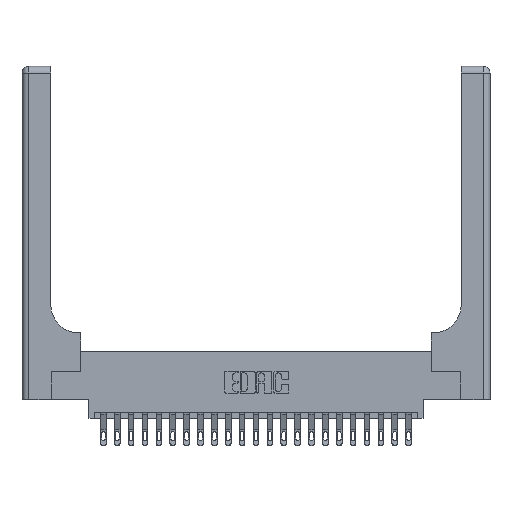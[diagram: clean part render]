
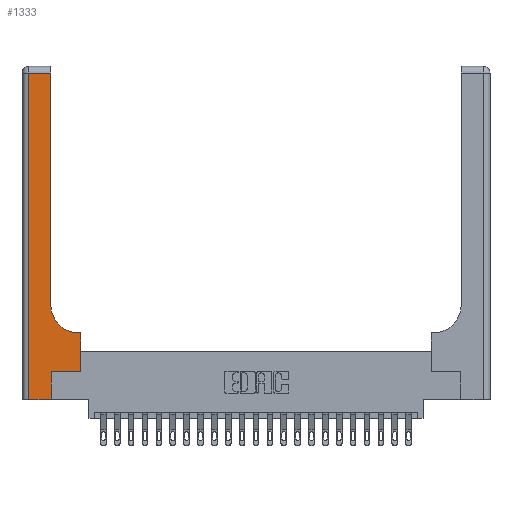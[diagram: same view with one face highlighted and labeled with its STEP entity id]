
A CAD part, top view. The second image highlights one B-rep face of the part: STEP entity #1333.
In plain terms, the highlighted planar face has unit normal (0, 0, 1).
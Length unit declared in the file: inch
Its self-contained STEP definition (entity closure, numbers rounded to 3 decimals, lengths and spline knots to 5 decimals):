
#25 = LINE ( 'NONE', #5152, #17082 ) ;
#84 = DIRECTION ( 'NONE',  ( 1., 0., 0. ) ) ;
#110 = LINE ( 'NONE', #20098, #6773 ) ;
#643 = CARTESIAN_POINT ( 'NONE',  ( 0.528, 0.25, 0.37 ) ) ;
#686 = ORIENTED_EDGE ( 'NONE', *, *, #16151, .T. ) ;
#844 = CIRCLE ( 'NONE', #3919, 0.25 ) ;
#1333 = ADVANCED_FACE ( 'NONE', ( #3418 ), #7256, .F. ) ;
#1612 = VECTOR ( 'NONE', #8010, 39.37008 ) ;
#1890 = LINE ( 'NONE', #9058, #10090 ) ;
#2270 = CARTESIAN_POINT ( 'NONE',  ( 0.265, 0.25, 0.37 ) ) ;
#2502 = EDGE_CURVE ( 'NONE', #13793, #22451, #25, .T. ) ;
#2514 = DIRECTION ( 'NONE',  ( -1., 0., 0. ) ) ;
#2807 = ORIENTED_EDGE ( 'NONE', *, *, #15712, .T. ) ;
#3418 = FACE_OUTER_BOUND ( 'NONE', #17989, .T. ) ;
#3423 = CARTESIAN_POINT ( 'NONE',  ( 0.06, 2.94, 0.37 ) ) ;
#3919 = AXIS2_PLACEMENT_3D ( 'NONE', #5829, #12874, #11330 ) ;
#4860 = EDGE_CURVE ( 'NONE', #4939, #21680, #1890, .T. ) ;
#4939 = VERTEX_POINT ( 'NONE', #22476 ) ;
#5152 = CARTESIAN_POINT ( 'NONE',  ( 0.528, 0.25, 0.37 ) ) ;
#5524 = DIRECTION ( 'NONE',  ( 0., 1., 0. ) ) ;
#5829 = CARTESIAN_POINT ( 'NONE',  ( 0.51, 0.85, 0.37 ) ) ;
#6468 = EDGE_CURVE ( 'NONE', #11177, #17295, #20722, .T. ) ;
#6472 = EDGE_CURVE ( 'NONE', #17295, #4939, #20365, .T. ) ;
#6773 = VECTOR ( 'NONE', #12912, 39.37008 ) ;
#7256 = PLANE ( 'NONE',  #18261 ) ;
#7475 = VERTEX_POINT ( 'NONE', #12216 ) ;
#7649 = LINE ( 'NONE', #2270, #1612 ) ;
#8010 = DIRECTION ( 'NONE',  ( 1., 0., 0. ) ) ;
#8067 = ORIENTED_EDGE ( 'NONE', *, *, #2502, .T. ) ;
#8995 = EDGE_CURVE ( 'NONE', #22451, #20019, #14100, .T. ) ;
#9058 = CARTESIAN_POINT ( 'NONE',  ( 0., 0., 0.37 ) ) ;
#9462 = CARTESIAN_POINT ( 'NONE',  ( 0., 2.94, 0.37 ) ) ;
#10090 = VECTOR ( 'NONE', #84, 39.37008 ) ;
#10317 = EDGE_CURVE ( 'NONE', #11606, #11177, #110, .T. ) ;
#10387 = CARTESIAN_POINT ( 'NONE',  ( 0.26, 0.6, 0.37 ) ) ;
#10578 = ORIENTED_EDGE ( 'NONE', *, *, #10317, .T. ) ;
#10715 = CARTESIAN_POINT ( 'NONE',  ( 0., 3., 0.37 ) ) ;
#11159 = ORIENTED_EDGE ( 'NONE', *, *, #23072, .T. ) ;
#11177 = VERTEX_POINT ( 'NONE', #16520 ) ;
#11330 = DIRECTION ( 'NONE',  ( 1., 0., 0. ) ) ;
#11606 = VERTEX_POINT ( 'NONE', #12433 ) ;
#12216 = CARTESIAN_POINT ( 'NONE',  ( 0.265, 0.25, 0.37 ) ) ;
#12433 = CARTESIAN_POINT ( 'NONE',  ( 0.26, 0.85, 0.37 ) ) ;
#12826 = ORIENTED_EDGE ( 'NONE', *, *, #6468, .T. ) ;
#12874 = DIRECTION ( 'NONE',  ( 0., 0., -1. ) ) ;
#12876 = VECTOR ( 'NONE', #17917, 39.37008 ) ;
#12912 = DIRECTION ( 'NONE',  ( 0., 1., 0. ) ) ;
#13793 = VERTEX_POINT ( 'NONE', #643 ) ;
#13967 = ORIENTED_EDGE ( 'NONE', *, *, #6472, .T. ) ;
#14100 = LINE ( 'NONE', #10387, #12876 ) ;
#14185 = DIRECTION ( 'NONE',  ( -1., 0., 0. ) ) ;
#14962 = CARTESIAN_POINT ( 'NONE',  ( 0.06, 3., 0.37 ) ) ;
#15482 = CARTESIAN_POINT ( 'NONE',  ( 0.265, 0., 0.37 ) ) ;
#15712 = EDGE_CURVE ( 'NONE', #7475, #13793, #7649, .T. ) ;
#15933 = CARTESIAN_POINT ( 'NONE',  ( 0.528, 0.6, 0.37 ) ) ;
#16151 = EDGE_CURVE ( 'NONE', #20019, #11606, #844, .T. ) ;
#16197 = DIRECTION ( 'NONE',  ( 0., 0., -1. ) ) ;
#16520 = CARTESIAN_POINT ( 'NONE',  ( 0.26, 2.94, 0.37 ) ) ;
#16868 = DIRECTION ( 'NONE',  ( 0., -1., 0. ) ) ;
#17082 = VECTOR ( 'NONE', #5524, 39.37008 ) ;
#17295 = VERTEX_POINT ( 'NONE', #3423 ) ;
#17896 = LINE ( 'NONE', #23177, #22478 ) ;
#17917 = DIRECTION ( 'NONE',  ( -1., 0., 0. ) ) ;
#17989 = EDGE_LOOP ( 'NONE', ( #10578, #12826, #13967, #19133, #11159, #2807, #8067, #22197, #686 ) ) ;
#18261 = AXIS2_PLACEMENT_3D ( 'NONE', #10715, #16197, #14185 ) ;
#19117 = VECTOR ( 'NONE', #2514, 39.37008 ) ;
#19133 = ORIENTED_EDGE ( 'NONE', *, *, #4860, .T. ) ;
#19951 = DIRECTION ( 'NONE',  ( 0., 1., 0. ) ) ;
#20019 = VERTEX_POINT ( 'NONE', #20703 ) ;
#20098 = CARTESIAN_POINT ( 'NONE',  ( 0.26, 3., 0.37 ) ) ;
#20365 = LINE ( 'NONE', #14962, #22956 ) ;
#20703 = CARTESIAN_POINT ( 'NONE',  ( 0.51, 0.6, 0.37 ) ) ;
#20722 = LINE ( 'NONE', #9462, #19117 ) ;
#21680 = VERTEX_POINT ( 'NONE', #15482 ) ;
#22197 = ORIENTED_EDGE ( 'NONE', *, *, #8995, .T. ) ;
#22451 = VERTEX_POINT ( 'NONE', #15933 ) ;
#22476 = CARTESIAN_POINT ( 'NONE',  ( 0.06, 0., 0.37 ) ) ;
#22478 = VECTOR ( 'NONE', #19951, 39.37008 ) ;
#22956 = VECTOR ( 'NONE', #16868, 39.37008 ) ;
#23072 = EDGE_CURVE ( 'NONE', #21680, #7475, #17896, .T. ) ;
#23177 = CARTESIAN_POINT ( 'NONE',  ( 0.265, 0., 0.37 ) ) ;
